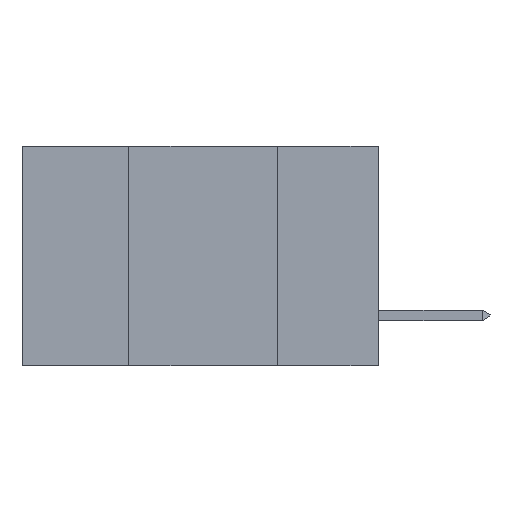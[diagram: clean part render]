
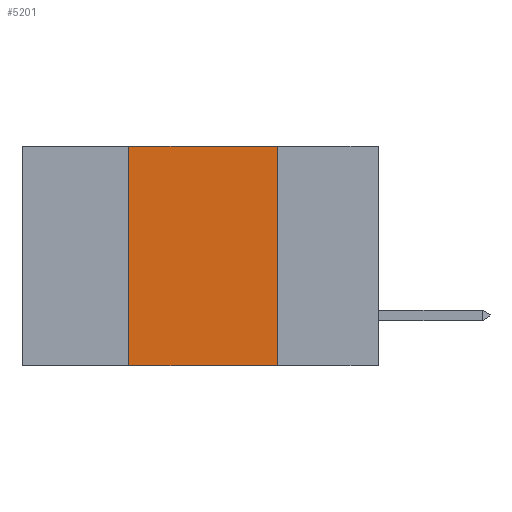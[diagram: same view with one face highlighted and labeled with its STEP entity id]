
A CAD part, left-side view. The second image highlights one B-rep face of the part: STEP entity #5201.
In plain terms, the highlighted planar face has unit normal (-1, 0, 0).
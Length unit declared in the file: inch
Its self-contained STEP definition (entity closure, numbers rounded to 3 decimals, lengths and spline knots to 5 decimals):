
#17 = LINE ( 'NONE', #9749, #6626 ) ;
#472 = DIRECTION ( 'NONE',  ( 0., 0., -1. ) ) ;
#1008 = VERTEX_POINT ( 'NONE', #4904 ) ;
#1371 = ORIENTED_EDGE ( 'NONE', *, *, #11409, .F. ) ;
#2377 = CARTESIAN_POINT ( 'NONE',  ( 0., 0.6, -0.37 ) ) ;
#3158 = LINE ( 'NONE', #2377, #6767 ) ;
#3170 = CARTESIAN_POINT ( 'NONE',  ( 0., 0.17, -0.37 ) ) ;
#3365 = PLANE ( 'NONE',  #9834 ) ;
#3540 = DIRECTION ( 'NONE',  ( 0., 0., -1. ) ) ;
#4500 = CARTESIAN_POINT ( 'NONE',  ( 0., 0.17, 0. ) ) ;
#4551 = DIRECTION ( 'NONE',  ( 0., 0., 1. ) ) ;
#4862 = VERTEX_POINT ( 'NONE', #8440 ) ;
#4884 = DIRECTION ( 'NONE',  ( 0., -1., 0. ) ) ;
#4904 = CARTESIAN_POINT ( 'NONE',  ( 0., 0.42, 0. ) ) ;
#5065 = ORIENTED_EDGE ( 'NONE', *, *, #8758, .F. ) ;
#5201 = ADVANCED_FACE ( 'NONE', ( #5333 ), #3365, .F. ) ;
#5333 = FACE_OUTER_BOUND ( 'NONE', #6250, .T. ) ;
#5687 = EDGE_CURVE ( 'NONE', #11110, #11877, #11393, .T. ) ;
#6250 = EDGE_LOOP ( 'NONE', ( #6380, #1371, #5065, #8009 ) ) ;
#6280 = DIRECTION ( 'NONE',  ( 0., -1., 0. ) ) ;
#6380 = ORIENTED_EDGE ( 'NONE', *, *, #5687, .F. ) ;
#6626 = VECTOR ( 'NONE', #4884, 39.37008 ) ;
#6767 = VECTOR ( 'NONE', #6280, 39.37008 ) ;
#7092 = EDGE_CURVE ( 'NONE', #4862, #11877, #3158, .T. ) ;
#7521 = LINE ( 'NONE', #9589, #8412 ) ;
#7549 = CARTESIAN_POINT ( 'NONE',  ( 0., 0.17, -0.37 ) ) ;
#8009 = ORIENTED_EDGE ( 'NONE', *, *, #7092, .T. ) ;
#8412 = VECTOR ( 'NONE', #4551, 39.37008 ) ;
#8440 = CARTESIAN_POINT ( 'NONE',  ( 0., 0.42, -0.37 ) ) ;
#8758 = EDGE_CURVE ( 'NONE', #4862, #1008, #7521, .T. ) ;
#9589 = CARTESIAN_POINT ( 'NONE',  ( 0., 0.42, -0.37 ) ) ;
#9749 = CARTESIAN_POINT ( 'NONE',  ( 0., 0.6, 0. ) ) ;
#9784 = CARTESIAN_POINT ( 'NONE',  ( 0., 0.6, 0. ) ) ;
#9834 = AXIS2_PLACEMENT_3D ( 'NONE', #9784, #9908, #472 ) ;
#9842 = VECTOR ( 'NONE', #3540, 39.37008 ) ;
#9908 = DIRECTION ( 'NONE',  ( 1., 0., 0. ) ) ;
#11110 = VERTEX_POINT ( 'NONE', #4500 ) ;
#11393 = LINE ( 'NONE', #7549, #9842 ) ;
#11409 = EDGE_CURVE ( 'NONE', #1008, #11110, #17, .T. ) ;
#11877 = VERTEX_POINT ( 'NONE', #3170 ) ;
